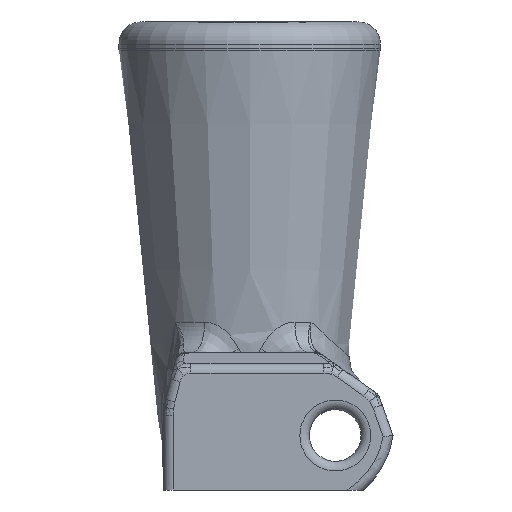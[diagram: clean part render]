
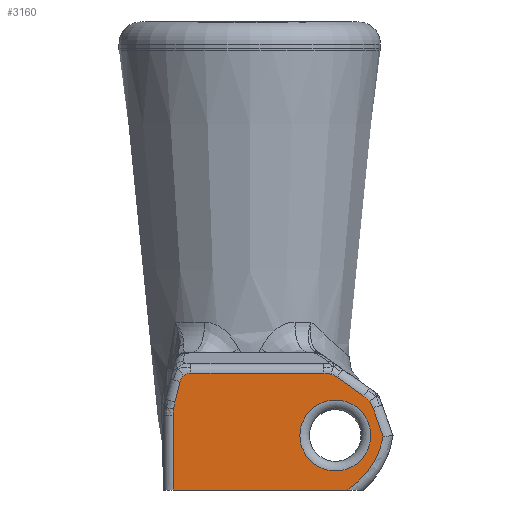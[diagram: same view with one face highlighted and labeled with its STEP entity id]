
A CAD part, left-side view. The second image highlights one B-rep face of the part: STEP entity #3160.
In plain terms, the highlighted planar face has unit normal (-1, 0, 0).
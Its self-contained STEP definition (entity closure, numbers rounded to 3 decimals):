
#42=FACE_BOUND('',#628,.T.);
#58=PLANE('',#3445);
#127=LINE('',#7437,#236);
#128=LINE('',#7439,#237);
#129=LINE('',#7442,#238);
#130=LINE('',#7443,#239);
#131=LINE('',#7444,#240);
#132=LINE('',#7445,#241);
#236=VECTOR('',#3949,10.);
#237=VECTOR('',#3950,10.);
#238=VECTOR('',#3953,10.);
#239=VECTOR('',#3954,10.);
#240=VECTOR('',#3955,10.);
#241=VECTOR('',#3956,10.);
#423=FACE_OUTER_BOUND('',#627,.T.);
#627=EDGE_LOOP('',(#2244,#2245,#2246,#2247,#2248,#2249,#2250,#2251,#2252,
#2253,#2254,#2255,#2256,#2257,#2258));
#628=EDGE_LOOP('',(#2259));
#784=CIRCLE('',#3317,4.118);
#787=CIRCLE('',#3320,4.118);
#790=CIRCLE('',#3323,0.808);
#793=CIRCLE('',#3326,0.808);
#804=CIRCLE('',#3337,1.695);
#807=CIRCLE('',#3340,1.695);
#830=CIRCLE('',#3363,1.789);
#833=CIRCLE('',#3366,1.789);
#902=CIRCLE('',#3439,2.575);
#907=CIRCLE('',#3446,5.667);
#1179=VERTEX_POINT('',#4653);
#1180=VERTEX_POINT('',#4660);
#1182=VERTEX_POINT('',#4706);
#1187=VERTEX_POINT('',#4799);
#1188=VERTEX_POINT('',#4806);
#1190=VERTEX_POINT('',#4852);
#1203=VERTEX_POINT('',#5129);
#1204=VERTEX_POINT('',#5136);
#1206=VERTEX_POINT('',#5182);
#1235=VERTEX_POINT('',#5751);
#1236=VERTEX_POINT('',#5758);
#1238=VERTEX_POINT('',#5804);
#1321=VERTEX_POINT('',#7424);
#1325=VERTEX_POINT('',#7436);
#1326=VERTEX_POINT('',#7438);
#1327=VERTEX_POINT('',#7440);
#1487=EDGE_CURVE('',#1179,#1180,#784,.T.);
#1491=EDGE_CURVE('',#1182,#1179,#787,.T.);
#1497=EDGE_CURVE('',#1187,#1188,#790,.T.);
#1501=EDGE_CURVE('',#1190,#1187,#793,.T.);
#1519=EDGE_CURVE('',#1203,#1204,#804,.T.);
#1523=EDGE_CURVE('',#1206,#1203,#807,.T.);
#1561=EDGE_CURVE('',#1235,#1236,#830,.T.);
#1565=EDGE_CURVE('',#1238,#1235,#833,.T.);
#1677=EDGE_CURVE('',#1321,#1321,#902,.T.);
#1683=EDGE_CURVE('',#1325,#1182,#127,.T.);
#1684=EDGE_CURVE('',#1326,#1325,#128,.T.);
#1685=EDGE_CURVE('',#1327,#1326,#907,.T.);
#1686=EDGE_CURVE('',#1236,#1327,#129,.T.);
#1687=EDGE_CURVE('',#1204,#1238,#130,.T.);
#1688=EDGE_CURVE('',#1188,#1206,#131,.T.);
#1689=EDGE_CURVE('',#1180,#1190,#132,.T.);
#2244=ORIENTED_EDGE('',*,*,#1683,.F.);
#2245=ORIENTED_EDGE('',*,*,#1684,.F.);
#2246=ORIENTED_EDGE('',*,*,#1685,.F.);
#2247=ORIENTED_EDGE('',*,*,#1686,.F.);
#2248=ORIENTED_EDGE('',*,*,#1561,.F.);
#2249=ORIENTED_EDGE('',*,*,#1565,.F.);
#2250=ORIENTED_EDGE('',*,*,#1687,.F.);
#2251=ORIENTED_EDGE('',*,*,#1519,.F.);
#2252=ORIENTED_EDGE('',*,*,#1523,.F.);
#2253=ORIENTED_EDGE('',*,*,#1688,.F.);
#2254=ORIENTED_EDGE('',*,*,#1497,.F.);
#2255=ORIENTED_EDGE('',*,*,#1501,.F.);
#2256=ORIENTED_EDGE('',*,*,#1689,.F.);
#2257=ORIENTED_EDGE('',*,*,#1487,.F.);
#2258=ORIENTED_EDGE('',*,*,#1491,.F.);
#2259=ORIENTED_EDGE('',*,*,#1677,.F.);
#3160=ADVANCED_FACE('',(#423,#42),#58,.T.);
#3317=AXIS2_PLACEMENT_3D('',#4661,#3688,#3689);
#3320=AXIS2_PLACEMENT_3D('',#4708,#3694,#3695);
#3323=AXIS2_PLACEMENT_3D('',#4807,#3700,#3701);
#3326=AXIS2_PLACEMENT_3D('',#4854,#3706,#3707);
#3337=AXIS2_PLACEMENT_3D('',#5137,#3728,#3729);
#3340=AXIS2_PLACEMENT_3D('',#5184,#3734,#3735);
#3363=AXIS2_PLACEMENT_3D('',#5759,#3780,#3781);
#3366=AXIS2_PLACEMENT_3D('',#5806,#3786,#3787);
#3439=AXIS2_PLACEMENT_3D('',#7425,#3934,#3935);
#3445=AXIS2_PLACEMENT_3D('',#7435,#3947,#3948);
#3446=AXIS2_PLACEMENT_3D('',#7441,#3951,#3952);
#3688=DIRECTION('center_axis',(1.,0.,0.));
#3689=DIRECTION('ref_axis',(0.,0.993,0.122));
#3694=DIRECTION('center_axis',(1.,0.,0.));
#3695=DIRECTION('ref_axis',(0.,0.993,0.122));
#3700=DIRECTION('center_axis',(1.,0.,0.));
#3701=DIRECTION('ref_axis',(0.,0.615,0.788));
#3706=DIRECTION('center_axis',(1.,0.,0.));
#3707=DIRECTION('ref_axis',(0.,0.615,0.788));
#3728=DIRECTION('center_axis',(1.,0.,0.));
#3729=DIRECTION('ref_axis',(0.,-0.302,0.953));
#3734=DIRECTION('center_axis',(1.,0.,0.));
#3735=DIRECTION('ref_axis',(0.,-0.302,0.953));
#3780=DIRECTION('center_axis',(1.,0.,0.));
#3781=DIRECTION('ref_axis',(0.,-0.795,0.606));
#3786=DIRECTION('center_axis',(1.,0.,0.));
#3787=DIRECTION('ref_axis',(0.,-0.795,0.606));
#3934=DIRECTION('center_axis',(-1.,0.,0.));
#3935=DIRECTION('ref_axis',(0.,1.,0.));
#3947=DIRECTION('center_axis',(-1.,0.,0.));
#3948=DIRECTION('ref_axis',(0.,-1.,0.));
#3949=DIRECTION('',(0.,0.,1.));
#3950=DIRECTION('',(0.,1.,0.));
#3951=DIRECTION('center_axis',(1.,0.,0.));
#3952=DIRECTION('ref_axis',(0.,-0.877,-0.48));
#3953=DIRECTION('',(0.,-0.338,-0.941));
#3954=DIRECTION('',(0.,-0.818,-0.575));
#3955=DIRECTION('',(0.,-1.,0.));
#3956=DIRECTION('',(0.,-0.243,0.97));
#4653=CARTESIAN_POINT('',(36.5,-44.481,12.26));
#4660=CARTESIAN_POINT('',(36.5,-44.573,12.756));
#4661=CARTESIAN_POINT('Origin',(36.5,-48.568,11.757));
#4706=CARTESIAN_POINT('',(36.5,-44.45,11.757));
#4708=CARTESIAN_POINT('Origin',(36.5,-48.568,11.757));
#4799=CARTESIAN_POINT('',(36.5,-45.229,14.674));
#4806=CARTESIAN_POINT('',(36.5,-45.726,14.845));
#4807=CARTESIAN_POINT('Origin',(36.5,-45.726,14.037));
#4852=CARTESIAN_POINT('',(36.5,-44.942,14.233));
#4854=CARTESIAN_POINT('Origin',(36.5,-45.726,14.037));
#5129=CARTESIAN_POINT('',(36.5,-55.897,14.766));
#5136=CARTESIAN_POINT('',(36.5,-56.361,14.537));
#5137=CARTESIAN_POINT('Origin',(36.5,-55.385,13.15));
#5182=CARTESIAN_POINT('',(36.5,-55.385,14.845));
#5184=CARTESIAN_POINT('Origin',(36.5,-55.385,13.15));
#5751=CARTESIAN_POINT('',(36.5,-58.694,12.793));
#5758=CARTESIAN_POINT('',(36.5,-58.955,12.313));
#5759=CARTESIAN_POINT('Origin',(36.5,-57.271,11.709));
#5804=CARTESIAN_POINT('',(36.5,-58.301,13.172));
#5806=CARTESIAN_POINT('Origin',(36.5,-57.271,11.709));
#7424=CARTESIAN_POINT('',(36.5,-56.217,12.885));
#7425=CARTESIAN_POINT('Origin',(36.5,-56.217,10.31));
#7435=CARTESIAN_POINT('Origin',(36.5,-41.75,6.35));
#7436=CARTESIAN_POINT('',(36.5,-44.45,6.35));
#7437=CARTESIAN_POINT('',(36.5,-44.45,6.35));
#7438=CARTESIAN_POINT('',(36.5,-57.062,6.35));
#7439=CARTESIAN_POINT('',(36.5,-58.25,6.35));
#7440=CARTESIAN_POINT('',(36.5,-59.698,10.241));
#7441=CARTESIAN_POINT('Origin',(36.5,-54.111,11.188));
#7442=CARTESIAN_POINT('',(36.5,-59.323,11.286));
#7443=CARTESIAN_POINT('',(36.5,-53.606,16.475));
#7444=CARTESIAN_POINT('',(36.5,-43.813,14.845));
#7445=CARTESIAN_POINT('',(36.5,-43.914,10.121));
